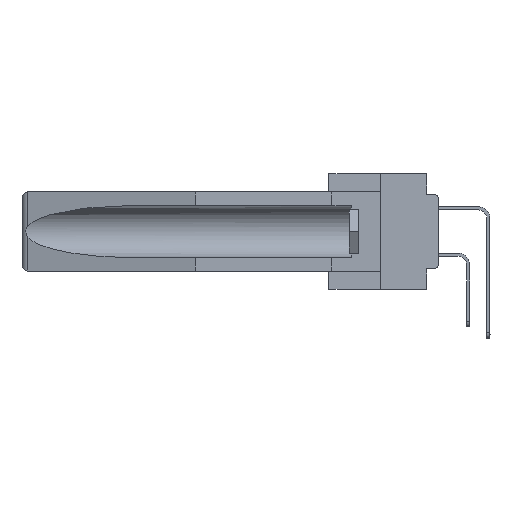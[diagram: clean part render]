
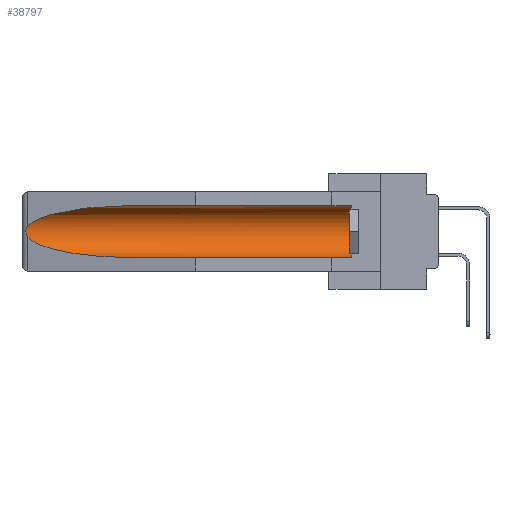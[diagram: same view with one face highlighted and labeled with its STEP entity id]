
A CAD part, left-side view. The second image highlights one B-rep face of the part: STEP entity #38797.
In plain terms, the highlighted cylindrical face has radius 2.857 mm (diameter 5.715 mm), a partial arc.
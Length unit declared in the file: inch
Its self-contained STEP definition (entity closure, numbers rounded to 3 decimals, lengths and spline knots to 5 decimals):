
#1738 = EDGE_CURVE ( 'NONE', #30608, #23016, #20185, .T. ) ;
#2377 = LINE ( 'NONE', #14433, #3782 ) ;
#3192 = CARTESIAN_POINT ( 'NONE',  ( 0.155, 1.07973, -0.284 ) ) ;
#3222 =( BOUNDED_CURVE ( )  B_SPLINE_CURVE ( 3, ( #17599, #14444, #26448, #14255 ),
 .UNSPECIFIED., .F., .F. ) 
 B_SPLINE_CURVE_WITH_KNOTS ( ( 4, 4 ),
 ( 4.71239, 6.08839 ),
 .UNSPECIFIED. ) 
 CURVE ( )  GEOMETRIC_REPRESENTATION_ITEM ( )  RATIONAL_B_SPLINE_CURVE ( ( 1., 0.848, 0.848, 1. ) ) 
 REPRESENTATION_ITEM ( '' )  );
#3628 = CARTESIAN_POINT ( 'NONE',  ( 0.155, -0.30754, -0.059 ) ) ;
#3782 = VECTOR ( 'NONE', #26641, 39.37008 ) ;
#4548 = ORIENTED_EDGE ( 'NONE', *, *, #1738, .T. ) ;
#4866 = CARTESIAN_POINT ( 'NONE',  ( 0.26654, 1.53092, -0.15636 ) ) ;
#5338 = EDGE_CURVE ( 'NONE', #23016, #14843, #12734, .T. ) ;
#6098 = CARTESIAN_POINT ( 'NONE',  ( 0.155, 1.07973, -0.059 ) ) ;
#6686 = CARTESIAN_POINT ( 'NONE',  ( 0.155, 0.126, -0.1715 ) ) ;
#6838 = AXIS2_PLACEMENT_3D ( 'NONE', #6686, #12232, #9077 ) ;
#6852 = CARTESIAN_POINT ( 'NONE',  ( 0.26537, 1.52718, -0.14972 ) ) ;
#6891 = DIRECTION ( 'NONE',  ( 0., 0., 1. ) ) ;
#7501 = EDGE_CURVE ( 'NONE', #25501, #22099, #24084, .T. ) ;
#8545 =( BOUNDED_CURVE ( )  B_SPLINE_CURVE ( 3, ( #25743, #13353, #16295, #25553 ),
 .UNSPECIFIED., .F., .F. ) 
 B_SPLINE_CURVE_WITH_KNOTS ( ( 4, 4 ),
 ( 0.1948, 1.5708 ),
 .UNSPECIFIED. ) 
 CURVE ( )  GEOMETRIC_REPRESENTATION_ITEM ( )  RATIONAL_B_SPLINE_CURVE ( ( 1., 0.848, 0.848, 1. ) ) 
 REPRESENTATION_ITEM ( '' )  );
#9077 = DIRECTION ( 'NONE',  ( 0., 0., 1. ) ) ;
#10511 = ORIENTED_EDGE ( 'NONE', *, *, #18434, .F. ) ;
#11717 = VECTOR ( 'NONE', #24749, 39.37008 ) ;
#12232 = DIRECTION ( 'NONE',  ( 0., -1., 0. ) ) ;
#12734 = LINE ( 'NONE', #3628, #11717 ) ;
#12826 = CARTESIAN_POINT ( 'NONE',  ( 0.155, -0.30754, -0.1715 ) ) ;
#13353 = CARTESIAN_POINT ( 'NONE',  ( 0.25451, 1.48313, -0.24835 ) ) ;
#14255 = CARTESIAN_POINT ( 'NONE',  ( 0.26537, 1.52718, -0.14972 ) ) ;
#14433 = CARTESIAN_POINT ( 'NONE',  ( 0.155, -0.30754, -0.284 ) ) ;
#14444 = CARTESIAN_POINT ( 'NONE',  ( 0.21114, 1.30732, -0.059 ) ) ;
#14843 = VERTEX_POINT ( 'NONE', #6098 ) ;
#15763 = DIRECTION ( 'NONE',  ( 0., 1., 0. ) ) ;
#16295 = CARTESIAN_POINT ( 'NONE',  ( 0.21114, 1.30732, -0.284 ) ) ;
#16528 = CARTESIAN_POINT ( 'NONE',  ( 0.26655, 1.53094, -0.18657 ) ) ;
#17599 = CARTESIAN_POINT ( 'NONE',  ( 0.155, 1.07973, -0.059 ) ) ;
#17723 = CARTESIAN_POINT ( 'NONE',  ( 0.155, 0.126, -0.284 ) ) ;
#18434 = EDGE_CURVE ( 'NONE', #30608, #29804, #2377, .T. ) ;
#18868 = ORIENTED_EDGE ( 'NONE', *, *, #21631, .T. ) ;
#19227 = CARTESIAN_POINT ( 'NONE',  ( 0.155, 0.126, -0.059 ) ) ;
#20185 = CIRCLE ( 'NONE', #6838, 0.1125 ) ;
#21631 = EDGE_CURVE ( 'NONE', #14843, #25501, #3222, .T. ) ;
#22099 = VERTEX_POINT ( 'NONE', #27330 ) ;
#22261 = AXIS2_PLACEMENT_3D ( 'NONE', #12826, #15763, #6891 ) ;
#22640 = CARTESIAN_POINT ( 'NONE',  ( 0.26597, 1.52961, -0.15275 ) ) ;
#23016 = VERTEX_POINT ( 'NONE', #19227 ) ;
#23583 = ORIENTED_EDGE ( 'NONE', *, *, #38099, .T. ) ;
#24084 = B_SPLINE_CURVE_WITH_KNOTS ( 'NONE', 3,
 ( #26161, #22640, #4866, #28916, #25776, #38007, #34277, #16528, #34856, #34462 ),
 .UNSPECIFIED., .F., .F.,
 ( 4, 2, 2, 2, 4 ),
 ( 0., 0.00029, 0.00058, 0.00087, 0.00117 ),
 .UNSPECIFIED. ) ;
#24749 = DIRECTION ( 'NONE',  ( 0., 1., 0. ) ) ;
#25501 = VERTEX_POINT ( 'NONE', #6852 ) ;
#25553 = CARTESIAN_POINT ( 'NONE',  ( 0.155, 1.07973, -0.284 ) ) ;
#25743 = CARTESIAN_POINT ( 'NONE',  ( 0.26537, 1.52718, -0.19328 ) ) ;
#25776 = CARTESIAN_POINT ( 'NONE',  ( 0.2675, 1.53308, -0.16763 ) ) ;
#26161 = CARTESIAN_POINT ( 'NONE',  ( 0.26537, 1.52718, -0.14972 ) ) ;
#26448 = CARTESIAN_POINT ( 'NONE',  ( 0.25451, 1.48313, -0.09465 ) ) ;
#26641 = DIRECTION ( 'NONE',  ( 0., 1., 0. ) ) ;
#27330 = CARTESIAN_POINT ( 'NONE',  ( 0.26537, 1.52718, -0.19328 ) ) ;
#28916 = CARTESIAN_POINT ( 'NONE',  ( 0.2673, 1.5327, -0.16383 ) ) ;
#29804 = VERTEX_POINT ( 'NONE', #3192 ) ;
#30608 = VERTEX_POINT ( 'NONE', #17723 ) ;
#30732 = FACE_OUTER_BOUND ( 'NONE', #37690, .T. ) ;
#30925 = CYLINDRICAL_SURFACE ( 'NONE', #22261, 0.1125 ) ;
#32812 = ORIENTED_EDGE ( 'NONE', *, *, #5338, .T. ) ;
#33225 = ORIENTED_EDGE ( 'NONE', *, *, #7501, .T. ) ;
#34277 = CARTESIAN_POINT ( 'NONE',  ( 0.2673, 1.53269, -0.17917 ) ) ;
#34462 = CARTESIAN_POINT ( 'NONE',  ( 0.26537, 1.52718, -0.19328 ) ) ;
#34856 = CARTESIAN_POINT ( 'NONE',  ( 0.26597, 1.5296, -0.19026 ) ) ;
#37690 = EDGE_LOOP ( 'NONE', ( #18868, #33225, #23583, #10511, #4548, #32812 ) ) ;
#38007 = CARTESIAN_POINT ( 'NONE',  ( 0.2675, 1.53308, -0.17534 ) ) ;
#38099 = EDGE_CURVE ( 'NONE', #22099, #29804, #8545, .T. ) ;
#38797 = ADVANCED_FACE ( 'NONE', ( #30732 ), #30925, .F. ) ;
